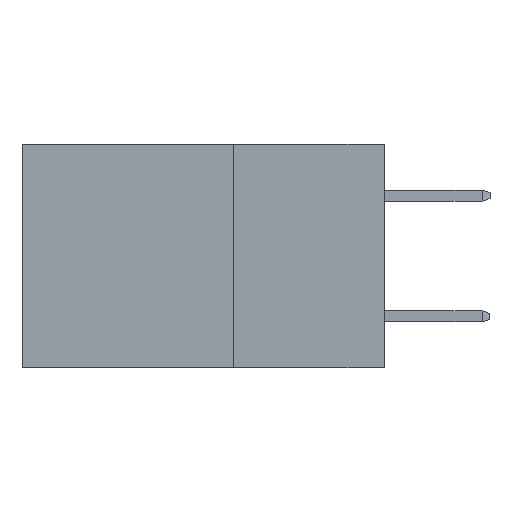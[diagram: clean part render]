
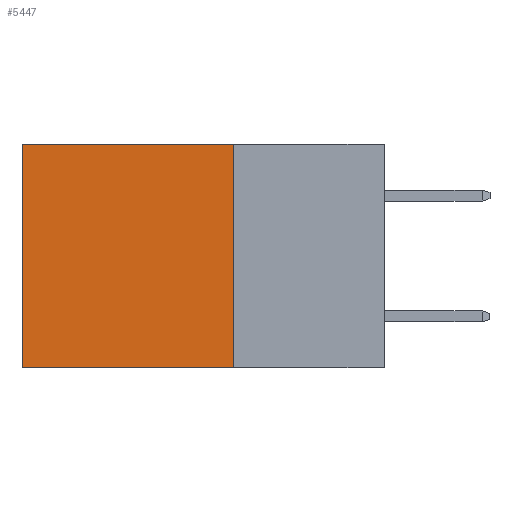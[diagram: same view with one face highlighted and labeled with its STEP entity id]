
A CAD part, left-side view. The second image highlights one B-rep face of the part: STEP entity #5447.
In plain terms, the highlighted planar face has unit normal (-1, 0, 0).
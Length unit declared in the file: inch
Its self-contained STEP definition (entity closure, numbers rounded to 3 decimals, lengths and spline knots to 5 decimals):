
#1175 = EDGE_CURVE ( 'NONE', #4288, #11193, #4035, .T. ) ;
#1741 = CARTESIAN_POINT ( 'NONE',  ( 0.298, 0.25, 0. ) ) ;
#1824 = CARTESIAN_POINT ( 'NONE',  ( 0.298, 0.25, -0.37 ) ) ;
#1825 = PLANE ( 'NONE',  #8805 ) ;
#2626 = ORIENTED_EDGE ( 'NONE', *, *, #6591, .F. ) ;
#2870 = CARTESIAN_POINT ( 'NONE',  ( 0.298, 0.25, 0. ) ) ;
#3050 = DIRECTION ( 'NONE',  ( 1., 0., 0. ) ) ;
#3268 = LINE ( 'NONE', #1824, #8573 ) ;
#4035 = LINE ( 'NONE', #6812, #5055 ) ;
#4061 = DIRECTION ( 'NONE',  ( 0., 1., 0. ) ) ;
#4288 = VERTEX_POINT ( 'NONE', #1741 ) ;
#4337 = LINE ( 'NONE', #2870, #7169 ) ;
#4432 = CARTESIAN_POINT ( 'NONE',  ( 0.298, 0.6, -0.37 ) ) ;
#5055 = VECTOR ( 'NONE', #8691, 39.37008 ) ;
#5425 = VERTEX_POINT ( 'NONE', #4432 ) ;
#5447 = ADVANCED_FACE ( 'NONE', ( #7652 ), #1825, .F. ) ;
#5688 = EDGE_CURVE ( 'NONE', #4288, #9283, #4337, .T. ) ;
#6220 = DIRECTION ( 'NONE',  ( 0., 0., -1. ) ) ;
#6227 = ORIENTED_EDGE ( 'NONE', *, *, #5688, .F. ) ;
#6591 = EDGE_CURVE ( 'NONE', #9283, #5425, #3268, .T. ) ;
#6812 = CARTESIAN_POINT ( 'NONE',  ( 0.298, 0.25, 0. ) ) ;
#7062 = ORIENTED_EDGE ( 'NONE', *, *, #1175, .T. ) ;
#7071 = CARTESIAN_POINT ( 'NONE',  ( 0.298, 0.25, 0. ) ) ;
#7169 = VECTOR ( 'NONE', #6220, 39.37008 ) ;
#7480 = DIRECTION ( 'NONE',  ( 0., 0., -1. ) ) ;
#7652 = FACE_OUTER_BOUND ( 'NONE', #9588, .T. ) ;
#8067 = VECTOR ( 'NONE', #8150, 39.37008 ) ;
#8150 = DIRECTION ( 'NONE',  ( 0., 0., -1. ) ) ;
#8552 = CARTESIAN_POINT ( 'NONE',  ( 0.298, 0.25, -0.37 ) ) ;
#8573 = VECTOR ( 'NONE', #4061, 39.37008 ) ;
#8691 = DIRECTION ( 'NONE',  ( 0., 1., 0. ) ) ;
#8805 = AXIS2_PLACEMENT_3D ( 'NONE', #7071, #3050, #7480 ) ;
#9283 = VERTEX_POINT ( 'NONE', #8552 ) ;
#9588 = EDGE_LOOP ( 'NONE', ( #10519, #2626, #6227, #7062 ) ) ;
#10519 = ORIENTED_EDGE ( 'NONE', *, *, #12291, .T. ) ;
#11131 = LINE ( 'NONE', #13372, #8067 ) ;
#11193 = VERTEX_POINT ( 'NONE', #11432 ) ;
#11432 = CARTESIAN_POINT ( 'NONE',  ( 0.298, 0.6, 0. ) ) ;
#12291 = EDGE_CURVE ( 'NONE', #11193, #5425, #11131, .T. ) ;
#13372 = CARTESIAN_POINT ( 'NONE',  ( 0.298, 0.6, 0. ) ) ;
